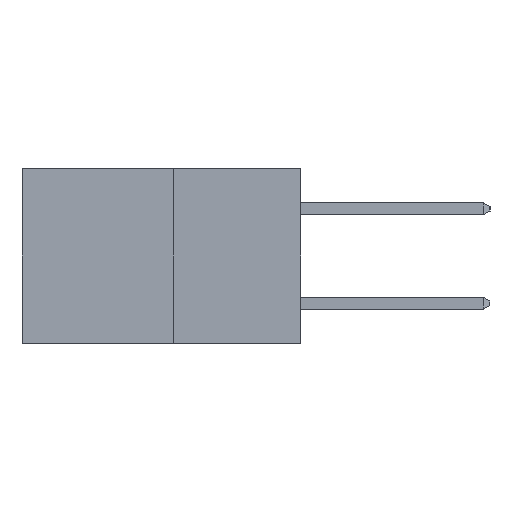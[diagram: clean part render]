
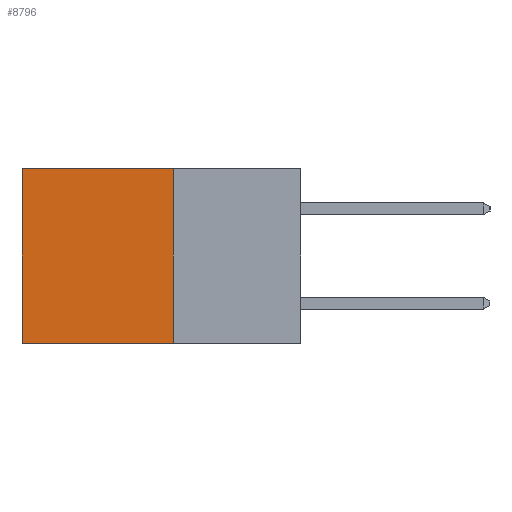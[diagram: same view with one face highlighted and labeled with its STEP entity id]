
A CAD part, left-side view. The second image highlights one B-rep face of the part: STEP entity #8796.
In plain terms, the highlighted planar face has unit normal (-1, 0, 0).
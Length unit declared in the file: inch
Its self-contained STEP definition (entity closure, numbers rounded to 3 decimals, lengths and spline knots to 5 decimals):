
#124 = VERTEX_POINT ( 'NONE', #4487 ) ;
#235 = VERTEX_POINT ( 'NONE', #7822 ) ;
#507 = CARTESIAN_POINT ( 'NONE',  ( 0.277, 0.27, -0.37 ) ) ;
#963 = EDGE_CURVE ( 'NONE', #235, #8835, #981, .T. ) ;
#981 = LINE ( 'NONE', #8884, #2435 ) ;
#1237 = CARTESIAN_POINT ( 'NONE',  ( 0.277, 0.27, -0.37 ) ) ;
#1951 = DIRECTION ( 'NONE',  ( 0., 0., -1. ) ) ;
#2224 = FACE_OUTER_BOUND ( 'NONE', #3980, .T. ) ;
#2435 = VECTOR ( 'NONE', #8913, 39.37008 ) ;
#2748 = VECTOR ( 'NONE', #8108, 39.37008 ) ;
#3098 = EDGE_CURVE ( 'NONE', #8835, #124, #7373, .T. ) ;
#3536 = ORIENTED_EDGE ( 'NONE', *, *, #7754, .T. ) ;
#3556 = ORIENTED_EDGE ( 'NONE', *, *, #7010, .T. ) ;
#3580 = CARTESIAN_POINT ( 'NONE',  ( 0.277, 0.59, 0. ) ) ;
#3872 = ORIENTED_EDGE ( 'NONE', *, *, #963, .F. ) ;
#3980 = EDGE_LOOP ( 'NONE', ( #3536, #4500, #3872, #3556 ) ) ;
#4399 = AXIS2_PLACEMENT_3D ( 'NONE', #1237, #6416, #1951 ) ;
#4487 = CARTESIAN_POINT ( 'NONE',  ( 0.277, 0.59, -0.37 ) ) ;
#4500 = ORIENTED_EDGE ( 'NONE', *, *, #3098, .F. ) ;
#4976 = VECTOR ( 'NONE', #9162, 39.37008 ) ;
#5565 = VERTEX_POINT ( 'NONE', #3580 ) ;
#5597 = CARTESIAN_POINT ( 'NONE',  ( 0.277, 0.59, -0.37 ) ) ;
#5642 = VECTOR ( 'NONE', #8303, 39.37008 ) ;
#5862 = LINE ( 'NONE', #7598, #5642 ) ;
#6416 = DIRECTION ( 'NONE',  ( 1., 0., 0. ) ) ;
#6881 = LINE ( 'NONE', #5597, #4976 ) ;
#7010 = EDGE_CURVE ( 'NONE', #235, #5565, #5862, .T. ) ;
#7373 = LINE ( 'NONE', #8830, #2748 ) ;
#7598 = CARTESIAN_POINT ( 'NONE',  ( 0.277, 0.27, 0. ) ) ;
#7754 = EDGE_CURVE ( 'NONE', #5565, #124, #6881, .T. ) ;
#7787 = PLANE ( 'NONE',  #4399 ) ;
#7822 = CARTESIAN_POINT ( 'NONE',  ( 0.277, 0.27, 0. ) ) ;
#8108 = DIRECTION ( 'NONE',  ( 0., 1., 0. ) ) ;
#8303 = DIRECTION ( 'NONE',  ( 0., 1., 0. ) ) ;
#8796 = ADVANCED_FACE ( 'NONE', ( #2224 ), #7787, .F. ) ;
#8830 = CARTESIAN_POINT ( 'NONE',  ( 0.277, 0.27, -0.37 ) ) ;
#8835 = VERTEX_POINT ( 'NONE', #507 ) ;
#8884 = CARTESIAN_POINT ( 'NONE',  ( 0.277, 0.27, -0.37 ) ) ;
#8913 = DIRECTION ( 'NONE',  ( 0., 0., -1. ) ) ;
#9162 = DIRECTION ( 'NONE',  ( 0., 0., -1. ) ) ;
